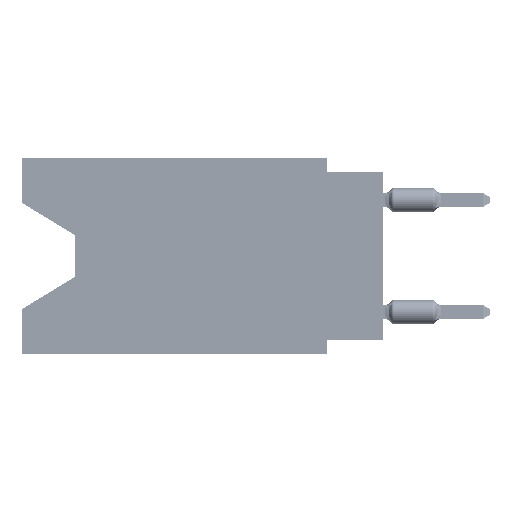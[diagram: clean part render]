
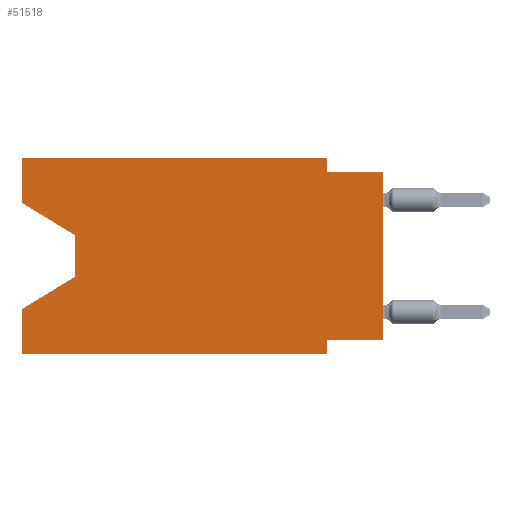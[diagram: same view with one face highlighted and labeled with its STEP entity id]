
A CAD part, left-side view. The second image highlights one B-rep face of the part: STEP entity #51518.
In plain terms, the highlighted planar face has unit normal (-1, 0, 0).
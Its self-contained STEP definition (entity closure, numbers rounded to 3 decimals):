
#1683 = VERTEX_POINT ( 'NONE', #64528 ) ;
#2377 = ORIENTED_EDGE ( 'NONE', *, *, #48170, .F. ) ;
#2886 = EDGE_CURVE ( 'NONE', #16858, #42963, #42837, .T. ) ;
#3659 = CARTESIAN_POINT ( 'NONE',  ( 0., 16.383, 0. ) ) ;
#3687 = EDGE_CURVE ( 'NONE', #15548, #19629, #19401, .T. ) ;
#3931 = VERTEX_POINT ( 'NONE', #60818 ) ;
#6515 = LINE ( 'NONE', #65232, #53698 ) ;
#6852 = CARTESIAN_POINT ( 'NONE',  ( 0., 16.383, -8.89 ) ) ;
#6856 = CARTESIAN_POINT ( 'NONE',  ( 0., 2.54, -8.255 ) ) ;
#6944 = VECTOR ( 'NONE', #24343, 1000. ) ;
#7046 = LINE ( 'NONE', #65763, #20941 ) ;
#9431 = DIRECTION ( 'NONE',  ( 0., 0., -1. ) ) ;
#10126 = VECTOR ( 'NONE', #68783, 1000. ) ;
#10961 = DIRECTION ( 'NONE',  ( 0., -1., 0. ) ) ;
#12258 = DIRECTION ( 'NONE',  ( 0., 0., -1. ) ) ;
#14450 = CARTESIAN_POINT ( 'NONE',  ( 0., 0., -8.255 ) ) ;
#14716 = LINE ( 'NONE', #57607, #50327 ) ;
#14743 = VECTOR ( 'NONE', #27701, 1000. ) ;
#15389 = ORIENTED_EDGE ( 'NONE', *, *, #3687, .F. ) ;
#15548 = VERTEX_POINT ( 'NONE', #6856 ) ;
#16477 = ORIENTED_EDGE ( 'NONE', *, *, #60352, .F. ) ;
#16858 = VERTEX_POINT ( 'NONE', #51133 ) ;
#17184 = AXIS2_PLACEMENT_3D ( 'NONE', #44917, #60411, #12258 ) ;
#18724 = LINE ( 'NONE', #34561, #6944 ) ;
#18832 = ORIENTED_EDGE ( 'NONE', *, *, #28863, .F. ) ;
#19401 = LINE ( 'NONE', #30652, #20353 ) ;
#19629 = VERTEX_POINT ( 'NONE', #19655 ) ;
#19655 = CARTESIAN_POINT ( 'NONE',  ( 0., 2.54, -8.89 ) ) ;
#19934 = LINE ( 'NONE', #41387, #10126 ) ;
#20353 = VECTOR ( 'NONE', #40854, 1000. ) ;
#20941 = VECTOR ( 'NONE', #29184, 1000. ) ;
#24343 = DIRECTION ( 'NONE',  ( 0., 0.855, -0.519 ) ) ;
#25265 = CARTESIAN_POINT ( 'NONE',  ( 0., 16.383, -2.038 ) ) ;
#25329 = DIRECTION ( 'NONE',  ( 0., -1., 0. ) ) ;
#25374 = VECTOR ( 'NONE', #66978, 1000. ) ;
#26336 = VERTEX_POINT ( 'NONE', #29158 ) ;
#27114 = VERTEX_POINT ( 'NONE', #6852 ) ;
#27701 = DIRECTION ( 'NONE',  ( 0., -1., 0. ) ) ;
#28740 = CARTESIAN_POINT ( 'NONE',  ( 0., 0., -8.255 ) ) ;
#28863 = EDGE_CURVE ( 'NONE', #29544, #42169, #63292, .T. ) ;
#29020 = CARTESIAN_POINT ( 'NONE',  ( 0., 13.97, -3.505 ) ) ;
#29158 = CARTESIAN_POINT ( 'NONE',  ( 0., 2.54, 0. ) ) ;
#29184 = DIRECTION ( 'NONE',  ( 0., 0., 1. ) ) ;
#29544 = VERTEX_POINT ( 'NONE', #51189 ) ;
#30077 = ORIENTED_EDGE ( 'NONE', *, *, #37145, .F. ) ;
#30652 = CARTESIAN_POINT ( 'NONE',  ( 0., 2.54, -8.89 ) ) ;
#31072 = EDGE_CURVE ( 'NONE', #48006, #42169, #6515, .T. ) ;
#32669 = ORIENTED_EDGE ( 'NONE', *, *, #37027, .F. ) ;
#34287 = VECTOR ( 'NONE', #40814, 1000. ) ;
#34561 = CARTESIAN_POINT ( 'NONE',  ( 0., 13.97, -5.385 ) ) ;
#36054 = EDGE_CURVE ( 'NONE', #48006, #15548, #51703, .T. ) ;
#36981 = LINE ( 'NONE', #64734, #44472 ) ;
#37027 = EDGE_CURVE ( 'NONE', #49146, #26336, #36981, .T. ) ;
#37145 = EDGE_CURVE ( 'NONE', #27114, #1683, #7046, .T. ) ;
#37918 = LINE ( 'NONE', #54771, #14743 ) ;
#38207 = LINE ( 'NONE', #29020, #25374 ) ;
#38887 = VECTOR ( 'NONE', #25329, 1000. ) ;
#38971 = FACE_OUTER_BOUND ( 'NONE', #58113, .T. ) ;
#40814 = DIRECTION ( 'NONE',  ( 0., 1., 0. ) ) ;
#40854 = DIRECTION ( 'NONE',  ( 0., 0., -1. ) ) ;
#41387 = CARTESIAN_POINT ( 'NONE',  ( 0., 16.383, 0. ) ) ;
#41645 = VECTOR ( 'NONE', #69208, 1000. ) ;
#42169 = VERTEX_POINT ( 'NONE', #67931 ) ;
#42837 = LINE ( 'NONE', #25265, #41645 ) ;
#42963 = VERTEX_POINT ( 'NONE', #49178 ) ;
#43386 = EDGE_CURVE ( 'NONE', #42963, #3931, #38207, .T. ) ;
#44472 = VECTOR ( 'NONE', #10961, 1000. ) ;
#44917 = CARTESIAN_POINT ( 'NONE',  ( 0., 16.383, 0. ) ) ;
#46324 = ORIENTED_EDGE ( 'NONE', *, *, #51854, .T. ) ;
#48006 = VERTEX_POINT ( 'NONE', #28740 ) ;
#48170 = EDGE_CURVE ( 'NONE', #16858, #49146, #19934, .T. ) ;
#49146 = VERTEX_POINT ( 'NONE', #3659 ) ;
#49178 = CARTESIAN_POINT ( 'NONE',  ( 0., 13.97, -3.505 ) ) ;
#49937 = ORIENTED_EDGE ( 'NONE', *, *, #2886, .T. ) ;
#50202 = PLANE ( 'NONE',  #17184 ) ;
#50327 = VECTOR ( 'NONE', #9431, 1000. ) ;
#51133 = CARTESIAN_POINT ( 'NONE',  ( 0., 16.383, -2.038 ) ) ;
#51189 = CARTESIAN_POINT ( 'NONE',  ( 0., 2.54, -0.635 ) ) ;
#51518 = ADVANCED_FACE ( 'NONE', ( #38971 ), #50202, .F. ) ;
#51703 = LINE ( 'NONE', #14450, #34287 ) ;
#51854 = EDGE_CURVE ( 'NONE', #3931, #1683, #18724, .T. ) ;
#52760 = CARTESIAN_POINT ( 'NONE',  ( 0., 0., -0.635 ) ) ;
#53075 = ORIENTED_EDGE ( 'NONE', *, *, #43386, .T. ) ;
#53655 = DIRECTION ( 'NONE',  ( 0., 0., 1. ) ) ;
#53698 = VECTOR ( 'NONE', #53655, 1000. ) ;
#54771 = CARTESIAN_POINT ( 'NONE',  ( 0., 16.383, -8.89 ) ) ;
#56396 = ORIENTED_EDGE ( 'NONE', *, *, #36054, .F. ) ;
#57607 = CARTESIAN_POINT ( 'NONE',  ( 0., 2.54, 0. ) ) ;
#58113 = EDGE_LOOP ( 'NONE', ( #49937, #53075, #46324, #30077, #65206, #15389, #56396, #67601, #18832, #16477, #32669, #2377 ) ) ;
#60352 = EDGE_CURVE ( 'NONE', #26336, #29544, #14716, .T. ) ;
#60411 = DIRECTION ( 'NONE',  ( 1., 0., 0. ) ) ;
#60818 = CARTESIAN_POINT ( 'NONE',  ( 0., 13.97, -5.385 ) ) ;
#63292 = LINE ( 'NONE', #52760, #38887 ) ;
#63780 = EDGE_CURVE ( 'NONE', #27114, #19629, #37918, .T. ) ;
#64528 = CARTESIAN_POINT ( 'NONE',  ( 0., 16.383, -6.852 ) ) ;
#64734 = CARTESIAN_POINT ( 'NONE',  ( 0., 16.383, 0. ) ) ;
#65206 = ORIENTED_EDGE ( 'NONE', *, *, #63780, .T. ) ;
#65232 = CARTESIAN_POINT ( 'NONE',  ( 0., 0., 0. ) ) ;
#65763 = CARTESIAN_POINT ( 'NONE',  ( 0., 16.383, 0. ) ) ;
#66978 = DIRECTION ( 'NONE',  ( 0., 0., -1. ) ) ;
#67601 = ORIENTED_EDGE ( 'NONE', *, *, #31072, .T. ) ;
#67931 = CARTESIAN_POINT ( 'NONE',  ( 0., 0., -0.635 ) ) ;
#68783 = DIRECTION ( 'NONE',  ( 0., 0., 1. ) ) ;
#69208 = DIRECTION ( 'NONE',  ( 0., -0.855, -0.519 ) ) ;
